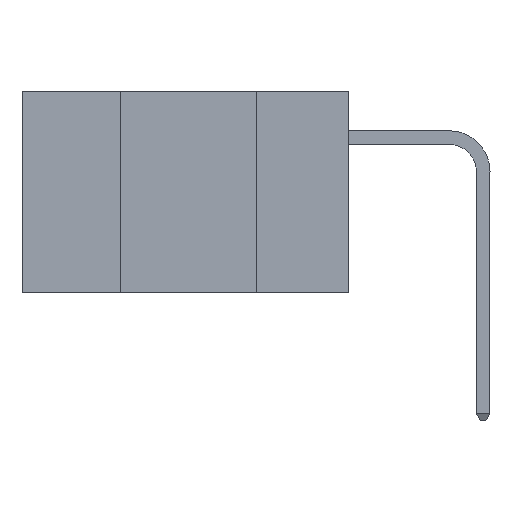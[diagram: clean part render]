
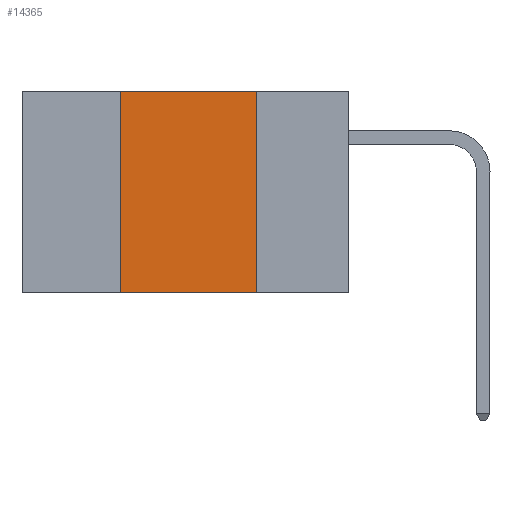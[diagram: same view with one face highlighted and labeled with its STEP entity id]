
A CAD part, left-side view. The second image highlights one B-rep face of the part: STEP entity #14365.
In plain terms, the highlighted planar face has unit normal (-1, 0, 0).
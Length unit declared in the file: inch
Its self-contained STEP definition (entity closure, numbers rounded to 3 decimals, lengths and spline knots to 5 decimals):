
#915 = VERTEX_POINT ( 'NONE', #17518 ) ;
#1665 = LINE ( 'NONE', #37035, #32867 ) ;
#2543 = CARTESIAN_POINT ( 'NONE',  ( 0., 0.6, 0. ) ) ;
#3032 = DIRECTION ( 'NONE',  ( 0., -1., 0. ) ) ;
#3192 = VECTOR ( 'NONE', #3032, 39.37008 ) ;
#3700 = VECTOR ( 'NONE', #38928, 39.37008 ) ;
#3719 = EDGE_CURVE ( 'NONE', #30459, #915, #35770, .T. ) ;
#4996 = EDGE_CURVE ( 'NONE', #8591, #21794, #1665, .T. ) ;
#7510 = DIRECTION ( 'NONE',  ( 0., -1., 0. ) ) ;
#8591 = VERTEX_POINT ( 'NONE', #10547 ) ;
#9715 = ORIENTED_EDGE ( 'NONE', *, *, #4996, .F. ) ;
#10094 = DIRECTION ( 'NONE',  ( 0., 0., -1. ) ) ;
#10213 = ORIENTED_EDGE ( 'NONE', *, *, #31438, .F. ) ;
#10374 = ORIENTED_EDGE ( 'NONE', *, *, #3719, .F. ) ;
#10481 = ORIENTED_EDGE ( 'NONE', *, *, #36257, .T. ) ;
#10547 = CARTESIAN_POINT ( 'NONE',  ( 0., 0.17, 0. ) ) ;
#11697 = PLANE ( 'NONE',  #34936 ) ;
#14365 = ADVANCED_FACE ( 'NONE', ( #30338 ), #11697, .F. ) ;
#14747 = DIRECTION ( 'NONE',  ( 0., 0., -1. ) ) ;
#16586 = EDGE_LOOP ( 'NONE', ( #9715, #10213, #10374, #10481 ) ) ;
#17518 = CARTESIAN_POINT ( 'NONE',  ( 0., 0.42, 0. ) ) ;
#19561 = CARTESIAN_POINT ( 'NONE',  ( 0., 0.6, -0.37 ) ) ;
#21055 = CARTESIAN_POINT ( 'NONE',  ( 0., 0.42, 0. ) ) ;
#21208 = CARTESIAN_POINT ( 'NONE',  ( 0., 0.6, 0. ) ) ;
#21503 = CARTESIAN_POINT ( 'NONE',  ( 0., 0.42, -0.37 ) ) ;
#21794 = VERTEX_POINT ( 'NONE', #29735 ) ;
#22288 = LINE ( 'NONE', #19561, #35373 ) ;
#26434 = LINE ( 'NONE', #21208, #3192 ) ;
#29735 = CARTESIAN_POINT ( 'NONE',  ( 0., 0.17, -0.37 ) ) ;
#30338 = FACE_OUTER_BOUND ( 'NONE', #16586, .T. ) ;
#30459 = VERTEX_POINT ( 'NONE', #21503 ) ;
#31438 = EDGE_CURVE ( 'NONE', #915, #8591, #26434, .T. ) ;
#32785 = DIRECTION ( 'NONE',  ( 1., 0., 0. ) ) ;
#32867 = VECTOR ( 'NONE', #10094, 39.37008 ) ;
#34936 = AXIS2_PLACEMENT_3D ( 'NONE', #2543, #32785, #14747 ) ;
#35373 = VECTOR ( 'NONE', #7510, 39.37008 ) ;
#35770 = LINE ( 'NONE', #21055, #3700 ) ;
#36257 = EDGE_CURVE ( 'NONE', #30459, #21794, #22288, .T. ) ;
#37035 = CARTESIAN_POINT ( 'NONE',  ( 0., 0.17, 0. ) ) ;
#38928 = DIRECTION ( 'NONE',  ( 0., 0., 1. ) ) ;
